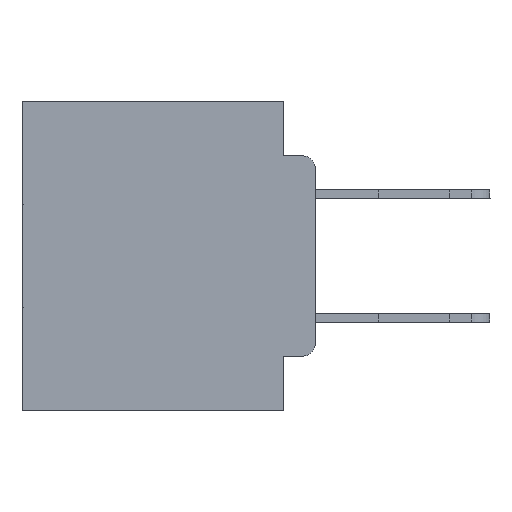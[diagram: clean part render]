
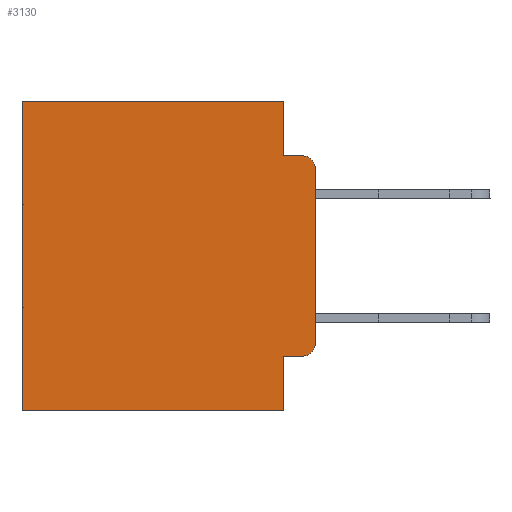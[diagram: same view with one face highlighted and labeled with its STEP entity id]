
A CAD part, left-side view. The second image highlights one B-rep face of the part: STEP entity #3130.
In plain terms, the highlighted planar face has unit normal (-1, 0, 0).
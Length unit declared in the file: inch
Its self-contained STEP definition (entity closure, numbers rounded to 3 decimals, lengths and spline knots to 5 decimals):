
#224 = EDGE_CURVE ( 'NONE', #6833, #29163, #29810, .T. ) ;
#478 = AXIS2_PLACEMENT_3D ( 'NONE', #19574, #5371, #21949 ) ;
#1155 = ORIENTED_EDGE ( 'NONE', *, *, #4980, .F. ) ;
#1212 = AXIS2_PLACEMENT_3D ( 'NONE', #9750, #26249, #12103 ) ;
#1690 = CARTESIAN_POINT ( 'NONE',  ( 0.298, 0.02, -0.4115 ) ) ;
#2016 = LINE ( 'NONE', #19117, #20197 ) ;
#2479 = CARTESIAN_POINT ( 'NONE',  ( 0.298, 0.051, 0. ) ) ;
#2685 = EDGE_CURVE ( 'NONE', #7033, #6833, #8779, .T. ) ;
#2751 = VERTEX_POINT ( 'NONE', #28261 ) ;
#2766 = CARTESIAN_POINT ( 'NONE',  ( 0.298, 0.051, -0.4115 ) ) ;
#3130 = ADVANCED_FACE ( 'NONE', ( #3192 ), #20336, .F. ) ;
#3192 = FACE_OUTER_BOUND ( 'NONE', #6316, .T. ) ;
#3378 = EDGE_CURVE ( 'NONE', #21701, #18862, #10277, .T. ) ;
#3399 = ORIENTED_EDGE ( 'NONE', *, *, #7567, .F. ) ;
#3781 = EDGE_CURVE ( 'NONE', #30509, #29163, #15807, .T. ) ;
#3944 = VECTOR ( 'NONE', #26926, 39.37008 ) ;
#4863 = DIRECTION ( 'NONE',  ( 0., 0., -1. ) ) ;
#4980 = EDGE_CURVE ( 'NONE', #21701, #30509, #2016, .T. ) ;
#5371 = DIRECTION ( 'NONE',  ( -1., 0., 0. ) ) ;
#5965 = ORIENTED_EDGE ( 'NONE', *, *, #3378, .T. ) ;
#6316 = EDGE_LOOP ( 'NONE', ( #3399, #15263, #8958, #10402, #28456, #15235, #26986, #1155, #5965, #17795 ) ) ;
#6833 = VERTEX_POINT ( 'NONE', #23104 ) ;
#7033 = VERTEX_POINT ( 'NONE', #26651 ) ;
#7567 = EDGE_CURVE ( 'NONE', #22602, #22289, #19664, .T. ) ;
#8779 = LINE ( 'NONE', #19704, #15829 ) ;
#8958 = ORIENTED_EDGE ( 'NONE', *, *, #16307, .F. ) ;
#9750 = CARTESIAN_POINT ( 'NONE',  ( 0.298, 0.02, -0.3915 ) ) ;
#10277 = LINE ( 'NONE', #11386, #26856 ) ;
#10402 = ORIENTED_EDGE ( 'NONE', *, *, #29235, .F. ) ;
#10626 = CIRCLE ( 'NONE', #1212, 0.02 ) ;
#11080 = VECTOR ( 'NONE', #4863, 39.37008 ) ;
#11127 = DIRECTION ( 'NONE',  ( 0., -1., 0. ) ) ;
#11386 = CARTESIAN_POINT ( 'NONE',  ( 0.298, 0.051, -0.4115 ) ) ;
#11680 = CARTESIAN_POINT ( 'NONE',  ( 0.298, 0.473, -0.5 ) ) ;
#12103 = DIRECTION ( 'NONE',  ( 0., 0., -1. ) ) ;
#13671 = AXIS2_PLACEMENT_3D ( 'NONE', #20515, #20233, #20203 ) ;
#13988 = CARTESIAN_POINT ( 'NONE',  ( 0.298, 0.051, -0.0885 ) ) ;
#14129 = DIRECTION ( 'NONE',  ( 0., 0., -1. ) ) ;
#15235 = ORIENTED_EDGE ( 'NONE', *, *, #224, .T. ) ;
#15263 = ORIENTED_EDGE ( 'NONE', *, *, #17431, .T. ) ;
#15807 = LINE ( 'NONE', #26962, #3944 ) ;
#15829 = VECTOR ( 'NONE', #29391, 39.37008 ) ;
#16187 = CARTESIAN_POINT ( 'NONE',  ( 0.298, 0.473, 0. ) ) ;
#16307 = EDGE_CURVE ( 'NONE', #18441, #2751, #21213, .T. ) ;
#17354 = VECTOR ( 'NONE', #17507, 39.37008 ) ;
#17382 = CARTESIAN_POINT ( 'NONE',  ( 0.298, 0., -0.3915 ) ) ;
#17431 = EDGE_CURVE ( 'NONE', #22602, #2751, #22237, .T. ) ;
#17507 = DIRECTION ( 'NONE',  ( 0., 0., -1. ) ) ;
#17795 = ORIENTED_EDGE ( 'NONE', *, *, #23921, .T. ) ;
#18441 = VERTEX_POINT ( 'NONE', #13988 ) ;
#18862 = VERTEX_POINT ( 'NONE', #1690 ) ;
#19117 = CARTESIAN_POINT ( 'NONE',  ( 0.298, 0.051, 0. ) ) ;
#19574 = CARTESIAN_POINT ( 'NONE',  ( 0.298, 0.02, -0.1085 ) ) ;
#19664 = LINE ( 'NONE', #28440, #11080 ) ;
#19704 = CARTESIAN_POINT ( 'NONE',  ( 0.298, 0., 0. ) ) ;
#19940 = DIRECTION ( 'NONE',  ( 0., -1., 0. ) ) ;
#20197 = VECTOR ( 'NONE', #14129, 39.37008 ) ;
#20203 = DIRECTION ( 'NONE',  ( 0., 0., -1. ) ) ;
#20233 = DIRECTION ( 'NONE',  ( 1., 0., 0. ) ) ;
#20336 = PLANE ( 'NONE',  #13671 ) ;
#20458 = VECTOR ( 'NONE', #19940, 39.37008 ) ;
#20515 = CARTESIAN_POINT ( 'NONE',  ( 0.298, 0., 0. ) ) ;
#21213 = LINE ( 'NONE', #26862, #20458 ) ;
#21460 = DIRECTION ( 'NONE',  ( 0., 0., -1. ) ) ;
#21701 = VERTEX_POINT ( 'NONE', #2766 ) ;
#21949 = DIRECTION ( 'NONE',  ( 0., 0., -1. ) ) ;
#22237 = CIRCLE ( 'NONE', #478, 0.02 ) ;
#22289 = VERTEX_POINT ( 'NONE', #17382 ) ;
#22602 = VERTEX_POINT ( 'NONE', #28023 ) ;
#22808 = CARTESIAN_POINT ( 'NONE',  ( 0.298, 0.051, -0.5 ) ) ;
#23104 = CARTESIAN_POINT ( 'NONE',  ( 0.298, 0.473, 0. ) ) ;
#23921 = EDGE_CURVE ( 'NONE', #18862, #22289, #10626, .T. ) ;
#25828 = VECTOR ( 'NONE', #21460, 39.37008 ) ;
#26249 = DIRECTION ( 'NONE',  ( -1., 0., 0. ) ) ;
#26557 = LINE ( 'NONE', #2479, #25828 ) ;
#26651 = CARTESIAN_POINT ( 'NONE',  ( 0.298, 0.051, 0. ) ) ;
#26856 = VECTOR ( 'NONE', #11127, 39.37008 ) ;
#26862 = CARTESIAN_POINT ( 'NONE',  ( 0.298, 0.051, -0.0885 ) ) ;
#26926 = DIRECTION ( 'NONE',  ( 0., 1., 0. ) ) ;
#26962 = CARTESIAN_POINT ( 'NONE',  ( 0.298, 0., -0.5 ) ) ;
#26986 = ORIENTED_EDGE ( 'NONE', *, *, #3781, .F. ) ;
#28023 = CARTESIAN_POINT ( 'NONE',  ( 0.298, 0., -0.1085 ) ) ;
#28261 = CARTESIAN_POINT ( 'NONE',  ( 0.298, 0.02, -0.0885 ) ) ;
#28440 = CARTESIAN_POINT ( 'NONE',  ( 0.298, 0., 0. ) ) ;
#28456 = ORIENTED_EDGE ( 'NONE', *, *, #2685, .T. ) ;
#29163 = VERTEX_POINT ( 'NONE', #11680 ) ;
#29235 = EDGE_CURVE ( 'NONE', #7033, #18441, #26557, .T. ) ;
#29391 = DIRECTION ( 'NONE',  ( 0., 1., 0. ) ) ;
#29810 = LINE ( 'NONE', #16187, #17354 ) ;
#30509 = VERTEX_POINT ( 'NONE', #22808 ) ;
